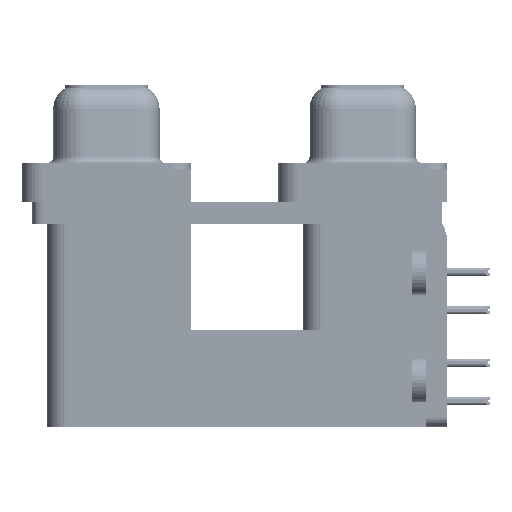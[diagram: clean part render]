
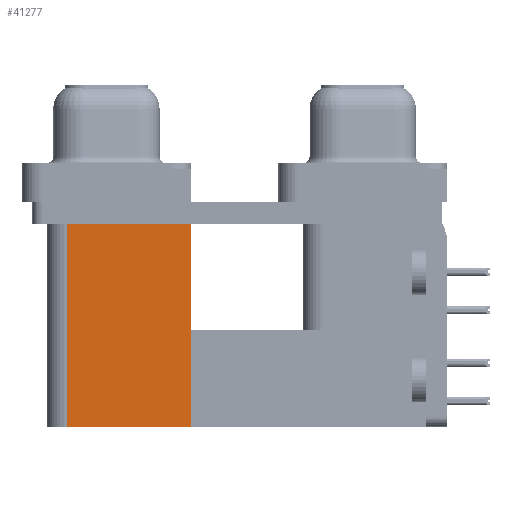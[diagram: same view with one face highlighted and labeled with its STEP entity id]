
A CAD part, left-side view. The second image highlights one B-rep face of the part: STEP entity #41277.
In plain terms, the highlighted planar face has unit normal (-1, 0, 0).
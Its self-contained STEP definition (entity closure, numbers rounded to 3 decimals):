
#5008 = CARTESIAN_POINT ( 'NONE',  ( 3.79, 12.775, -19.2 ) ) ;
#8477 = ORIENTED_EDGE ( 'NONE', *, *, #19145, .T. ) ;
#8756 = VERTEX_POINT ( 'NONE', #55707 ) ;
#9263 = PLANE ( 'NONE',  #65158 ) ;
#11552 = LINE ( 'NONE', #34537, #74241 ) ;
#14064 = CARTESIAN_POINT ( 'NONE',  ( 3.79, 21.975, -2.5 ) ) ;
#14534 = VERTEX_POINT ( 'NONE', #14064 ) ;
#18513 = CARTESIAN_POINT ( 'NONE',  ( 3.79, 21.975, -19.2 ) ) ;
#19145 = EDGE_CURVE ( 'NONE', #8756, #14534, #40535, .T. ) ;
#19467 = CARTESIAN_POINT ( 'NONE',  ( 3.79, 12.775, -19.2 ) ) ;
#22131 = EDGE_LOOP ( 'NONE', ( #8477, #43249, #71610, #52737 ) ) ;
#22796 = LINE ( 'NONE', #34845, #58932 ) ;
#23555 = EDGE_CURVE ( 'NONE', #65688, #8756, #38925, .T. ) ;
#28078 = DIRECTION ( 'NONE',  ( 0., 0., 1. ) ) ;
#28891 = DIRECTION ( 'NONE',  ( 0., 1., 0. ) ) ;
#34537 = CARTESIAN_POINT ( 'NONE',  ( 3.79, 12.775, -19.2 ) ) ;
#34845 = CARTESIAN_POINT ( 'NONE',  ( 3.79, 21.975, -19.2 ) ) ;
#38803 = EDGE_CURVE ( 'NONE', #58843, #14534, #22796, .T. ) ;
#38925 = LINE ( 'NONE', #5008, #69531 ) ;
#40535 = LINE ( 'NONE', #47294, #53412 ) ;
#40832 = CARTESIAN_POINT ( 'NONE',  ( 3.79, 12.775, -19.2 ) ) ;
#41277 = ADVANCED_FACE ( 'NONE', ( #65790 ), #9263, .F. ) ;
#42802 = DIRECTION ( 'NONE',  ( 0., 0., -1. ) ) ;
#43249 = ORIENTED_EDGE ( 'NONE', *, *, #38803, .F. ) ;
#47294 = CARTESIAN_POINT ( 'NONE',  ( 3.79, 12.775, -2.5 ) ) ;
#52737 = ORIENTED_EDGE ( 'NONE', *, *, #23555, .T. ) ;
#53412 = VECTOR ( 'NONE', #70272, 1000. ) ;
#55707 = CARTESIAN_POINT ( 'NONE',  ( 3.79, 12.775, -2.5 ) ) ;
#58462 = EDGE_CURVE ( 'NONE', #65688, #58843, #11552, .T. ) ;
#58843 = VERTEX_POINT ( 'NONE', #18513 ) ;
#58932 = VECTOR ( 'NONE', #28078, 1000. ) ;
#61924 = DIRECTION ( 'NONE',  ( 0., 0., 1. ) ) ;
#65158 = AXIS2_PLACEMENT_3D ( 'NONE', #19467, #66537, #42802 ) ;
#65688 = VERTEX_POINT ( 'NONE', #40832 ) ;
#65790 = FACE_OUTER_BOUND ( 'NONE', #22131, .T. ) ;
#66537 = DIRECTION ( 'NONE',  ( 1., 0., 0. ) ) ;
#69531 = VECTOR ( 'NONE', #61924, 1000. ) ;
#70272 = DIRECTION ( 'NONE',  ( 0., 1., 0. ) ) ;
#71610 = ORIENTED_EDGE ( 'NONE', *, *, #58462, .F. ) ;
#74241 = VECTOR ( 'NONE', #28891, 1000. ) ;
